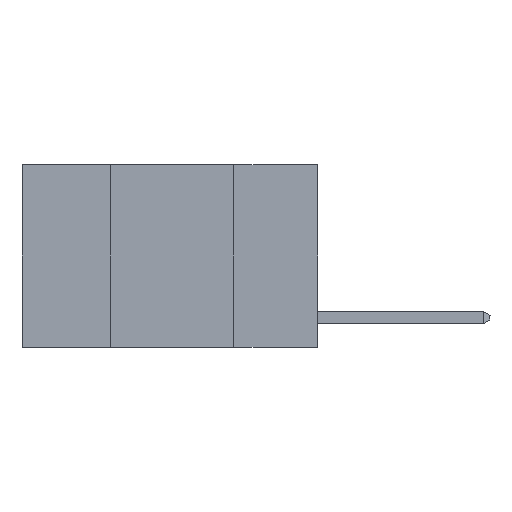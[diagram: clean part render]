
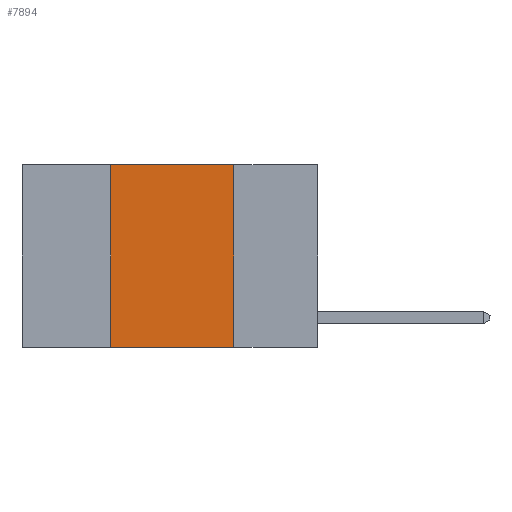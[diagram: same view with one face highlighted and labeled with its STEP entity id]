
A CAD part, left-side view. The second image highlights one B-rep face of the part: STEP entity #7894.
In plain terms, the highlighted planar face has unit normal (-1, 0, 0).
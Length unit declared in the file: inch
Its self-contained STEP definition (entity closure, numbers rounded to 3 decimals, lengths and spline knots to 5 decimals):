
#50 = CARTESIAN_POINT ( 'NONE',  ( 0., 0.42, -0.37 ) ) ;
#381 = FACE_OUTER_BOUND ( 'NONE', #11959, .T. ) ;
#1213 = VECTOR ( 'NONE', #7751, 39.37008 ) ;
#1232 = ORIENTED_EDGE ( 'NONE', *, *, #10222, .F. ) ;
#1298 = VECTOR ( 'NONE', #6713, 39.37008 ) ;
#1407 = CARTESIAN_POINT ( 'NONE',  ( 0., 0.6, 0. ) ) ;
#1670 = VECTOR ( 'NONE', #3963, 39.37008 ) ;
#3963 = DIRECTION ( 'NONE',  ( 0., -1., 0. ) ) ;
#4503 = VECTOR ( 'NONE', #13918, 39.37008 ) ;
#4725 = PLANE ( 'NONE',  #5656 ) ;
#4771 = VERTEX_POINT ( 'NONE', #9864 ) ;
#5005 = CARTESIAN_POINT ( 'NONE',  ( 0., 0.6, -0.37 ) ) ;
#5320 = VERTEX_POINT ( 'NONE', #50 ) ;
#5545 = LINE ( 'NONE', #10023, #1298 ) ;
#5656 = AXIS2_PLACEMENT_3D ( 'NONE', #1407, #7938, #5895 ) ;
#5895 = DIRECTION ( 'NONE',  ( 0., 0., -1. ) ) ;
#6656 = CARTESIAN_POINT ( 'NONE',  ( 0., 0.6, 0. ) ) ;
#6713 = DIRECTION ( 'NONE',  ( 0., 0., -1. ) ) ;
#6725 = ORIENTED_EDGE ( 'NONE', *, *, #9732, .T. ) ;
#7139 = ORIENTED_EDGE ( 'NONE', *, *, #9748, .F. ) ;
#7200 = LINE ( 'NONE', #7343, #4503 ) ;
#7343 = CARTESIAN_POINT ( 'NONE',  ( 0., 0.42, 0. ) ) ;
#7751 = DIRECTION ( 'NONE',  ( 0., -1., 0. ) ) ;
#7894 = ADVANCED_FACE ( 'NONE', ( #381 ), #4725, .F. ) ;
#7938 = DIRECTION ( 'NONE',  ( 1., 0., 0. ) ) ;
#8095 = VERTEX_POINT ( 'NONE', #11982 ) ;
#8451 = CARTESIAN_POINT ( 'NONE',  ( 0., 0.17, 0. ) ) ;
#9296 = VERTEX_POINT ( 'NONE', #8451 ) ;
#9531 = LINE ( 'NONE', #5005, #1670 ) ;
#9732 = EDGE_CURVE ( 'NONE', #5320, #4771, #9531, .T. ) ;
#9748 = EDGE_CURVE ( 'NONE', #5320, #8095, #7200, .T. ) ;
#9864 = CARTESIAN_POINT ( 'NONE',  ( 0., 0.17, -0.37 ) ) ;
#10023 = CARTESIAN_POINT ( 'NONE',  ( 0., 0.17, 0. ) ) ;
#10222 = EDGE_CURVE ( 'NONE', #8095, #9296, #13037, .T. ) ;
#11959 = EDGE_LOOP ( 'NONE', ( #13611, #1232, #7139, #6725 ) ) ;
#11982 = CARTESIAN_POINT ( 'NONE',  ( 0., 0.42, 0. ) ) ;
#13037 = LINE ( 'NONE', #6656, #1213 ) ;
#13611 = ORIENTED_EDGE ( 'NONE', *, *, #14247, .F. ) ;
#13918 = DIRECTION ( 'NONE',  ( 0., 0., 1. ) ) ;
#14247 = EDGE_CURVE ( 'NONE', #9296, #4771, #5545, .T. ) ;
